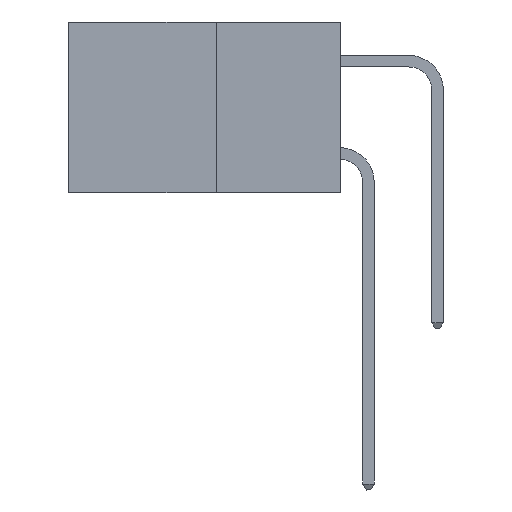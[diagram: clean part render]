
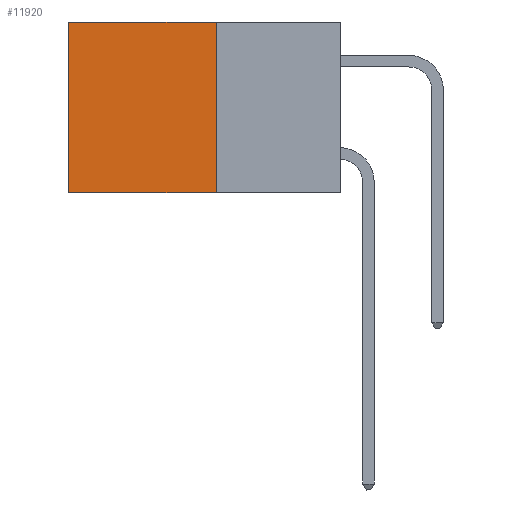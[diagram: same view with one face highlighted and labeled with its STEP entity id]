
A CAD part, left-side view. The second image highlights one B-rep face of the part: STEP entity #11920.
In plain terms, the highlighted planar face has unit normal (-1, 0, 0).
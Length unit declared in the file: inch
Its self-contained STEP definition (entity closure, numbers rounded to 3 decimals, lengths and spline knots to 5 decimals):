
#58 = VECTOR ( 'NONE', #4073, 39.37008 ) ;
#211 = CARTESIAN_POINT ( 'NONE',  ( 0.277, 0.27, -0.37 ) ) ;
#282 = CARTESIAN_POINT ( 'NONE',  ( 0.277, 0.59, -0.37 ) ) ;
#380 = VERTEX_POINT ( 'NONE', #1463 ) ;
#389 = CARTESIAN_POINT ( 'NONE',  ( 0.277, 0.27, 0. ) ) ;
#1306 = EDGE_CURVE ( 'NONE', #380, #2157, #11722, .T. ) ;
#1463 = CARTESIAN_POINT ( 'NONE',  ( 0.277, 0.27, -0.37 ) ) ;
#1733 = LINE ( 'NONE', #3063, #6731 ) ;
#2157 = VERTEX_POINT ( 'NONE', #282 ) ;
#2460 = CARTESIAN_POINT ( 'NONE',  ( 0.277, 0.59, 0. ) ) ;
#2599 = EDGE_CURVE ( 'NONE', #6772, #9623, #1733, .T. ) ;
#3063 = CARTESIAN_POINT ( 'NONE',  ( 0.277, 0.27, 0. ) ) ;
#3207 = EDGE_CURVE ( 'NONE', #6772, #380, #11496, .T. ) ;
#4073 = DIRECTION ( 'NONE',  ( 0., 1., 0. ) ) ;
#4390 = PLANE ( 'NONE',  #13113 ) ;
#4721 = LINE ( 'NONE', #8271, #7497 ) ;
#5544 = DIRECTION ( 'NONE',  ( 0., 0., -1. ) ) ;
#5864 = ORIENTED_EDGE ( 'NONE', *, *, #3207, .F. ) ;
#6731 = VECTOR ( 'NONE', #10662, 39.37008 ) ;
#6772 = VERTEX_POINT ( 'NONE', #389 ) ;
#7149 = DIRECTION ( 'NONE',  ( 0., 0., -1. ) ) ;
#7497 = VECTOR ( 'NONE', #7149, 39.37008 ) ;
#7883 = CARTESIAN_POINT ( 'NONE',  ( 0.277, 0.27, -0.37 ) ) ;
#8271 = CARTESIAN_POINT ( 'NONE',  ( 0.277, 0.59, -0.37 ) ) ;
#8545 = VECTOR ( 'NONE', #13901, 39.37008 ) ;
#8721 = FACE_OUTER_BOUND ( 'NONE', #12679, .T. ) ;
#9623 = VERTEX_POINT ( 'NONE', #2460 ) ;
#10662 = DIRECTION ( 'NONE',  ( 0., 1., 0. ) ) ;
#11247 = ORIENTED_EDGE ( 'NONE', *, *, #2599, .T. ) ;
#11496 = LINE ( 'NONE', #13944, #8545 ) ;
#11722 = LINE ( 'NONE', #211, #58 ) ;
#11920 = ADVANCED_FACE ( 'NONE', ( #8721 ), #4390, .F. ) ;
#12307 = DIRECTION ( 'NONE',  ( 1., 0., 0. ) ) ;
#12679 = EDGE_LOOP ( 'NONE', ( #13387, #13043, #5864, #11247 ) ) ;
#13043 = ORIENTED_EDGE ( 'NONE', *, *, #1306, .F. ) ;
#13113 = AXIS2_PLACEMENT_3D ( 'NONE', #7883, #12307, #5544 ) ;
#13387 = ORIENTED_EDGE ( 'NONE', *, *, #13873, .T. ) ;
#13873 = EDGE_CURVE ( 'NONE', #9623, #2157, #4721, .T. ) ;
#13901 = DIRECTION ( 'NONE',  ( 0., 0., -1. ) ) ;
#13944 = CARTESIAN_POINT ( 'NONE',  ( 0.277, 0.27, -0.37 ) ) ;
